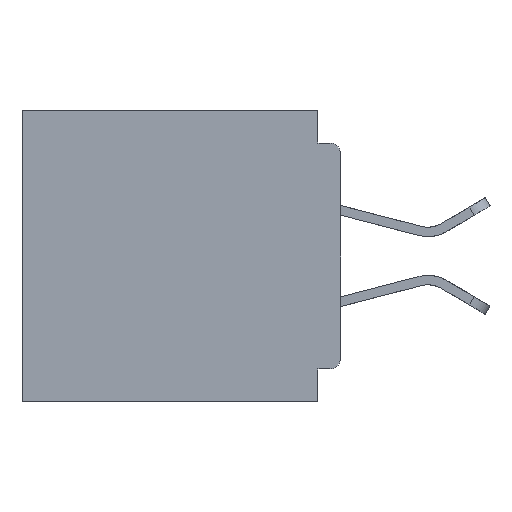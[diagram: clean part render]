
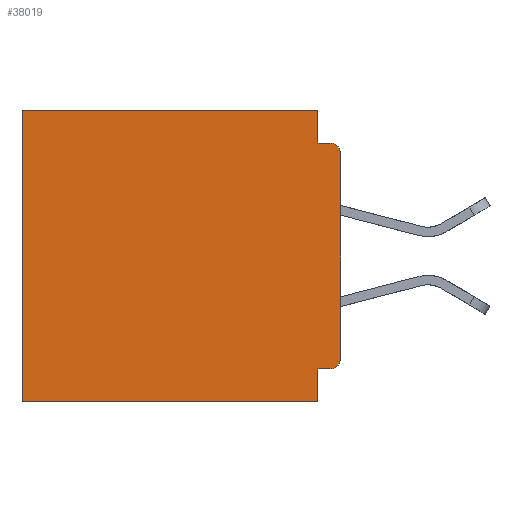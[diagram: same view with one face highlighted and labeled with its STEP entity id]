
A CAD part, left-side view. The second image highlights one B-rep face of the part: STEP entity #38019.
In plain terms, the highlighted planar face has unit normal (-1, 0, 0).
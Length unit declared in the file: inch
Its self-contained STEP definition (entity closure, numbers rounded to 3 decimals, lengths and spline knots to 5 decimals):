
#385 = ORIENTED_EDGE ( 'NONE', *, *, #33430, .F. ) ;
#572 = CARTESIAN_POINT ( 'NONE',  ( 0.3, 0.437, -0.4 ) ) ;
#697 = DIRECTION ( 'NONE',  ( 0., 0., -1. ) ) ;
#2344 = CARTESIAN_POINT ( 'NONE',  ( 0.3, 0., -0.045 ) ) ;
#2448 = VECTOR ( 'NONE', #29370, 39.37008 ) ;
#2746 = CARTESIAN_POINT ( 'NONE',  ( 0.3, 0.015, -0.06 ) ) ;
#4595 = EDGE_CURVE ( 'NONE', #27773, #9604, #25232, .T. ) ;
#4628 = CARTESIAN_POINT ( 'NONE',  ( 0.3, 0., -0.355 ) ) ;
#5230 = VERTEX_POINT ( 'NONE', #16631 ) ;
#5672 = CARTESIAN_POINT ( 'NONE',  ( 0.3, 0., -0.4 ) ) ;
#5845 = DIRECTION ( 'NONE',  ( 0., 0., -1. ) ) ;
#6381 = EDGE_CURVE ( 'NONE', #15418, #6719, #34826, .T. ) ;
#6550 = AXIS2_PLACEMENT_3D ( 'NONE', #2746, #23993, #5845 ) ;
#6719 = VERTEX_POINT ( 'NONE', #23837 ) ;
#6830 = AXIS2_PLACEMENT_3D ( 'NONE', #25168, #7033, #28181 ) ;
#7033 = DIRECTION ( 'NONE',  ( -1., 0., 0. ) ) ;
#7104 = ORIENTED_EDGE ( 'NONE', *, *, #4595, .F. ) ;
#7366 = VECTOR ( 'NONE', #32647, 39.37008 ) ;
#7430 = ORIENTED_EDGE ( 'NONE', *, *, #36169, .F. ) ;
#8306 = DIRECTION ( 'NONE',  ( 0., 0., -1. ) ) ;
#8529 = ORIENTED_EDGE ( 'NONE', *, *, #37432, .T. ) ;
#8537 = EDGE_LOOP ( 'NONE', ( #7430, #8529, #32283, #36438, #14247, #26333, #7104, #10816, #385, #27204 ) ) ;
#8774 = DIRECTION ( 'NONE',  ( 0., 0., -1. ) ) ;
#9043 = CIRCLE ( 'NONE', #6550, 0.015 ) ;
#9198 = VERTEX_POINT ( 'NONE', #10853 ) ;
#9604 = VERTEX_POINT ( 'NONE', #572 ) ;
#9674 = LINE ( 'NONE', #11373, #2448 ) ;
#10424 = FACE_OUTER_BOUND ( 'NONE', #8537, .T. ) ;
#10816 = ORIENTED_EDGE ( 'NONE', *, *, #24950, .F. ) ;
#10853 = CARTESIAN_POINT ( 'NONE',  ( 0.3, 0.015, -0.045 ) ) ;
#10995 = CARTESIAN_POINT ( 'NONE',  ( 0.3, 0., 0. ) ) ;
#11233 = AXIS2_PLACEMENT_3D ( 'NONE', #5672, #26839, #8774 ) ;
#11373 = CARTESIAN_POINT ( 'NONE',  ( 0.3, 0.437, -0.4 ) ) ;
#11693 = CARTESIAN_POINT ( 'NONE',  ( 0.3, 0.031, 0. ) ) ;
#13287 = EDGE_CURVE ( 'NONE', #35499, #9198, #17363, .T. ) ;
#14247 = ORIENTED_EDGE ( 'NONE', *, *, #38976, .T. ) ;
#14758 = PLANE ( 'NONE',  #11233 ) ;
#15226 = VERTEX_POINT ( 'NONE', #21221 ) ;
#15329 = LINE ( 'NONE', #22021, #23719 ) ;
#15418 = VERTEX_POINT ( 'NONE', #18962 ) ;
#16052 = LINE ( 'NONE', #4628, #17003 ) ;
#16631 = CARTESIAN_POINT ( 'NONE',  ( 0.3, 0., -0.06 ) ) ;
#17003 = VECTOR ( 'NONE', #28863, 39.37008 ) ;
#17238 = VECTOR ( 'NONE', #33905, 39.37008 ) ;
#17363 = LINE ( 'NONE', #2344, #7366 ) ;
#17584 = VERTEX_POINT ( 'NONE', #11693 ) ;
#18962 = CARTESIAN_POINT ( 'NONE',  ( 0.3, 0.015, -0.355 ) ) ;
#19296 = CARTESIAN_POINT ( 'NONE',  ( 0.3, 0.031, 0. ) ) ;
#20341 = CARTESIAN_POINT ( 'NONE',  ( 0.3, 0.031, -0.4 ) ) ;
#20483 = CARTESIAN_POINT ( 'NONE',  ( 0.3, 0., -0.4 ) ) ;
#20694 = VECTOR ( 'NONE', #8306, 39.37008 ) ;
#21221 = CARTESIAN_POINT ( 'NONE',  ( 0.3, 0.437, 0. ) ) ;
#21487 = VERTEX_POINT ( 'NONE', #29859 ) ;
#22021 = CARTESIAN_POINT ( 'NONE',  ( 0.3, 0., -0.4 ) ) ;
#22940 = EDGE_CURVE ( 'NONE', #17584, #35499, #33242, .T. ) ;
#23101 = DIRECTION ( 'NONE',  ( 0., 1., 0. ) ) ;
#23719 = VECTOR ( 'NONE', #697, 39.37008 ) ;
#23837 = CARTESIAN_POINT ( 'NONE',  ( 0.3, 0., -0.34 ) ) ;
#23993 = DIRECTION ( 'NONE',  ( -1., 0., 0. ) ) ;
#24950 = EDGE_CURVE ( 'NONE', #21487, #27773, #29604, .T. ) ;
#25168 = CARTESIAN_POINT ( 'NONE',  ( 0.3, 0.015, -0.34 ) ) ;
#25232 = LINE ( 'NONE', #20483, #17238 ) ;
#26333 = ORIENTED_EDGE ( 'NONE', *, *, #26852, .T. ) ;
#26839 = DIRECTION ( 'NONE',  ( 1., 0., 0. ) ) ;
#26852 = EDGE_CURVE ( 'NONE', #15226, #9604, #9674, .T. ) ;
#27204 = ORIENTED_EDGE ( 'NONE', *, *, #6381, .T. ) ;
#27773 = VERTEX_POINT ( 'NONE', #33738 ) ;
#28181 = DIRECTION ( 'NONE',  ( 0., 0., -1. ) ) ;
#28863 = DIRECTION ( 'NONE',  ( 0., 1., 0. ) ) ;
#29370 = DIRECTION ( 'NONE',  ( 0., 0., -1. ) ) ;
#29604 = LINE ( 'NONE', #20341, #20694 ) ;
#29859 = CARTESIAN_POINT ( 'NONE',  ( 0.3, 0.031, -0.355 ) ) ;
#31520 = LINE ( 'NONE', #10995, #38515 ) ;
#32283 = ORIENTED_EDGE ( 'NONE', *, *, #13287, .F. ) ;
#32308 = VECTOR ( 'NONE', #37252, 39.37008 ) ;
#32647 = DIRECTION ( 'NONE',  ( 0., -1., 0. ) ) ;
#33242 = LINE ( 'NONE', #19296, #32308 ) ;
#33430 = EDGE_CURVE ( 'NONE', #15418, #21487, #16052, .T. ) ;
#33738 = CARTESIAN_POINT ( 'NONE',  ( 0.3, 0.031, -0.4 ) ) ;
#33905 = DIRECTION ( 'NONE',  ( 0., 1., 0. ) ) ;
#34826 = CIRCLE ( 'NONE', #6830, 0.015 ) ;
#35499 = VERTEX_POINT ( 'NONE', #39052 ) ;
#36169 = EDGE_CURVE ( 'NONE', #5230, #6719, #15329, .T. ) ;
#36438 = ORIENTED_EDGE ( 'NONE', *, *, #22940, .F. ) ;
#37252 = DIRECTION ( 'NONE',  ( 0., 0., -1. ) ) ;
#37432 = EDGE_CURVE ( 'NONE', #5230, #9198, #9043, .T. ) ;
#38019 = ADVANCED_FACE ( 'NONE', ( #10424 ), #14758, .F. ) ;
#38515 = VECTOR ( 'NONE', #23101, 39.37008 ) ;
#38976 = EDGE_CURVE ( 'NONE', #17584, #15226, #31520, .T. ) ;
#39052 = CARTESIAN_POINT ( 'NONE',  ( 0.3, 0.031, -0.045 ) ) ;
